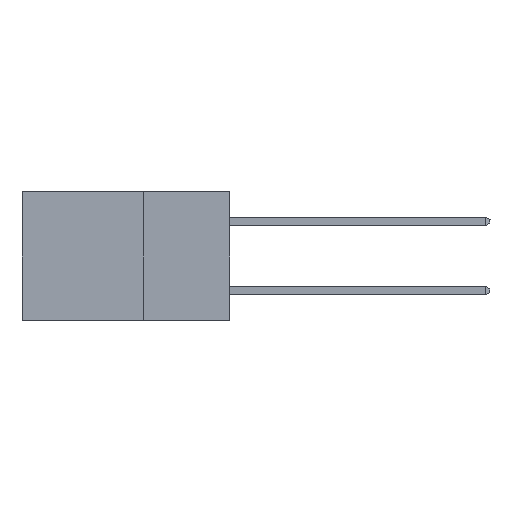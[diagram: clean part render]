
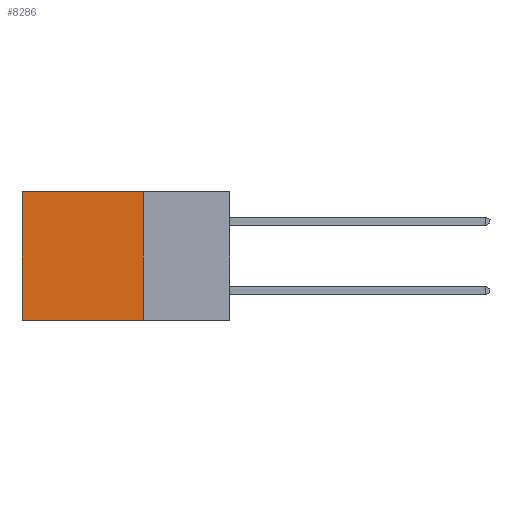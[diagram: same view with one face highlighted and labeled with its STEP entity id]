
A CAD part, left-side view. The second image highlights one B-rep face of the part: STEP entity #8286.
In plain terms, the highlighted planar face has unit normal (-1, 0, 0).
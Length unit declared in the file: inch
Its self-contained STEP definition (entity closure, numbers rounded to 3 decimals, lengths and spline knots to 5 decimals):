
#787 = ORIENTED_EDGE ( 'NONE', *, *, #9088, .F. ) ;
#912 = VECTOR ( 'NONE', #13297, 39.37008 ) ;
#1451 = EDGE_LOOP ( 'NONE', ( #7937, #787, #7747, #3443 ) ) ;
#1588 = VECTOR ( 'NONE', #8705, 39.37008 ) ;
#1874 = FACE_OUTER_BOUND ( 'NONE', #1451, .T. ) ;
#3126 = DIRECTION ( 'NONE',  ( 0., 0., -1. ) ) ;
#3286 = CARTESIAN_POINT ( 'NONE',  ( 0.2615, 0.6, 0. ) ) ;
#3443 = ORIENTED_EDGE ( 'NONE', *, *, #4427, .T. ) ;
#3670 = DIRECTION ( 'NONE',  ( 0., 1., 0. ) ) ;
#4408 = VERTEX_POINT ( 'NONE', #5867 ) ;
#4427 = EDGE_CURVE ( 'NONE', #12333, #6717, #8845, .T. ) ;
#4647 = CARTESIAN_POINT ( 'NONE',  ( 0.2615, 0.25, -0.37 ) ) ;
#4844 = DIRECTION ( 'NONE',  ( 1., 0., 0. ) ) ;
#5796 = CARTESIAN_POINT ( 'NONE',  ( 0.2615, 0.25, -0.37 ) ) ;
#5856 = PLANE ( 'NONE',  #8119 ) ;
#5867 = CARTESIAN_POINT ( 'NONE',  ( 0.2615, 0.6, -0.37 ) ) ;
#5916 = EDGE_CURVE ( 'NONE', #12333, #13230, #7556, .T. ) ;
#5935 = CARTESIAN_POINT ( 'NONE',  ( 0.2615, 0.25, 0. ) ) ;
#6717 = VERTEX_POINT ( 'NONE', #3286 ) ;
#7556 = LINE ( 'NONE', #4647, #1588 ) ;
#7589 = EDGE_CURVE ( 'NONE', #6717, #4408, #10409, .T. ) ;
#7747 = ORIENTED_EDGE ( 'NONE', *, *, #5916, .F. ) ;
#7937 = ORIENTED_EDGE ( 'NONE', *, *, #7589, .T. ) ;
#8119 = AXIS2_PLACEMENT_3D ( 'NONE', #5796, #4844, #9282 ) ;
#8286 = ADVANCED_FACE ( 'NONE', ( #1874 ), #5856, .F. ) ;
#8705 = DIRECTION ( 'NONE',  ( 0., 0., -1. ) ) ;
#8798 = LINE ( 'NONE', #12924, #10274 ) ;
#8845 = LINE ( 'NONE', #5935, #912 ) ;
#9088 = EDGE_CURVE ( 'NONE', #13230, #4408, #8798, .T. ) ;
#9282 = DIRECTION ( 'NONE',  ( 0., 0., -1. ) ) ;
#9467 = CARTESIAN_POINT ( 'NONE',  ( 0.2615, 0.6, -0.37 ) ) ;
#9764 = CARTESIAN_POINT ( 'NONE',  ( 0.2615, 0.25, -0.37 ) ) ;
#10274 = VECTOR ( 'NONE', #3670, 39.37008 ) ;
#10409 = LINE ( 'NONE', #9467, #10630 ) ;
#10630 = VECTOR ( 'NONE', #3126, 39.37008 ) ;
#12164 = CARTESIAN_POINT ( 'NONE',  ( 0.2615, 0.25, 0. ) ) ;
#12333 = VERTEX_POINT ( 'NONE', #12164 ) ;
#12924 = CARTESIAN_POINT ( 'NONE',  ( 0.2615, 0.25, -0.37 ) ) ;
#13230 = VERTEX_POINT ( 'NONE', #9764 ) ;
#13297 = DIRECTION ( 'NONE',  ( 0., 1., 0. ) ) ;
